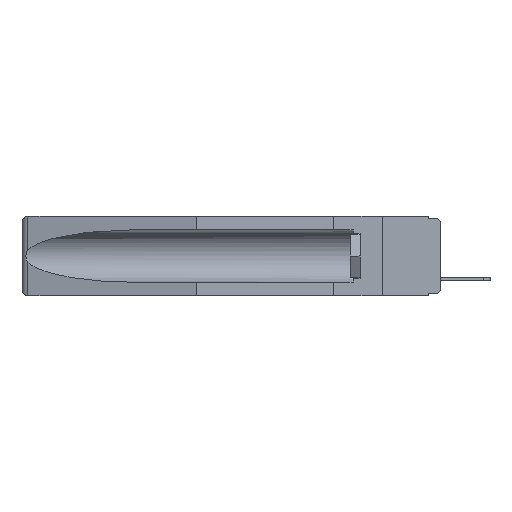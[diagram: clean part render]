
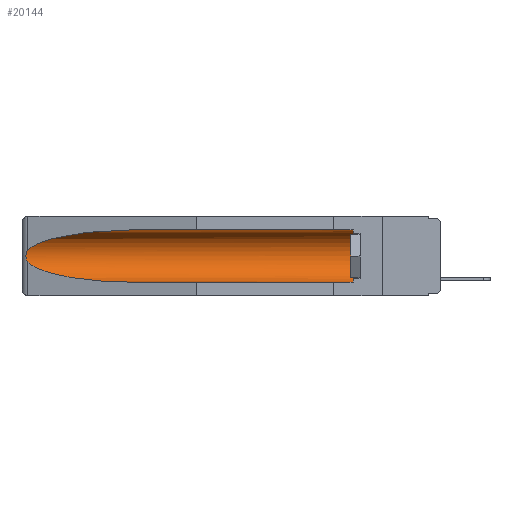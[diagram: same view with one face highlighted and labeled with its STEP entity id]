
A CAD part, left-side view. The second image highlights one B-rep face of the part: STEP entity #20144.
In plain terms, the highlighted cylindrical face has radius 2.857 mm (diameter 5.715 mm), a partial arc.
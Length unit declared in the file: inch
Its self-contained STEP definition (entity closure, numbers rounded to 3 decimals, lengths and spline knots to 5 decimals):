
#684 = DIRECTION ( 'NONE',  ( 0., 1., 0. ) ) ;
#697 = DIRECTION ( 'NONE',  ( 0., 1., 0. ) ) ;
#1230 = EDGE_CURVE ( 'NONE', #21232, #1581, #12304, .T. ) ;
#1581 = VERTEX_POINT ( 'NONE', #13792 ) ;
#2259 = AXIS2_PLACEMENT_3D ( 'NONE', #9138, #697, #20834 ) ;
#2445 = CARTESIAN_POINT ( 'NONE',  ( 0.155, -0.30754, -0.284 ) ) ;
#3760 = CARTESIAN_POINT ( 'NONE',  ( 0.155, 0.126, -0.1715 ) ) ;
#4679 = CARTESIAN_POINT ( 'NONE',  ( 0.2673, 1.5327, -0.16383 ) ) ;
#5197 = CARTESIAN_POINT ( 'NONE',  ( 0.26537, 1.52718, -0.14972 ) ) ;
#5404 = CARTESIAN_POINT ( 'NONE',  ( 0.21114, 1.30732, -0.059 ) ) ;
#5410 = VERTEX_POINT ( 'NONE', #13827 ) ;
#5419 = ORIENTED_EDGE ( 'NONE', *, *, #8624, .T. ) ;
#5649 = CARTESIAN_POINT ( 'NONE',  ( 0.26537, 1.52718, -0.19328 ) ) ;
#6218 = CARTESIAN_POINT ( 'NONE',  ( 0.26597, 1.52961, -0.15275 ) ) ;
#6237 = VERTEX_POINT ( 'NONE', #11287 ) ;
#6435 = CARTESIAN_POINT ( 'NONE',  ( 0.26655, 1.53094, -0.18657 ) ) ;
#7325 = EDGE_CURVE ( 'NONE', #20696, #21232, #14255, .T. ) ;
#7818 = ORIENTED_EDGE ( 'NONE', *, *, #16306, .T. ) ;
#7897 = CARTESIAN_POINT ( 'NONE',  ( 0.26537, 1.52718, -0.14972 ) ) ;
#8107 = CARTESIAN_POINT ( 'NONE',  ( 0.26537, 1.52718, -0.19328 ) ) ;
#8624 = EDGE_CURVE ( 'NONE', #11812, #5410, #18479, .T. ) ;
#8701 = ORIENTED_EDGE ( 'NONE', *, *, #7325, .T. ) ;
#8877 = CARTESIAN_POINT ( 'NONE',  ( 0.155, 1.07973, -0.284 ) ) ;
#9138 = CARTESIAN_POINT ( 'NONE',  ( 0.155, -0.30754, -0.1715 ) ) ;
#9272 = CARTESIAN_POINT ( 'NONE',  ( 0.155, -0.30754, -0.059 ) ) ;
#9832 = VECTOR ( 'NONE', #684, 39.37008 ) ;
#10224 = EDGE_LOOP ( 'NONE', ( #16617, #7818, #5419, #15835, #13134, #8701 ) ) ;
#11287 = CARTESIAN_POINT ( 'NONE',  ( 0.155, 0.126, -0.284 ) ) ;
#11518 = FACE_OUTER_BOUND ( 'NONE', #10224, .T. ) ;
#11812 = VERTEX_POINT ( 'NONE', #5649 ) ;
#12304 =( BOUNDED_CURVE ( )  B_SPLINE_CURVE ( 3, ( #18713, #5404, #17066, #5197 ),
 .UNSPECIFIED., .F., .F. ) 
 B_SPLINE_CURVE_WITH_KNOTS ( ( 4, 4 ),
 ( 4.71239, 6.08839 ),
 .UNSPECIFIED. ) 
 CURVE ( )  GEOMETRIC_REPRESENTATION_ITEM ( )  RATIONAL_B_SPLINE_CURVE ( ( 1., 0.848, 0.848, 1. ) ) 
 REPRESENTATION_ITEM ( '' )  );
#12768 = CARTESIAN_POINT ( 'NONE',  ( 0.155, 1.07973, -0.059 ) ) ;
#13134 = ORIENTED_EDGE ( 'NONE', *, *, #16993, .T. ) ;
#13758 = CIRCLE ( 'NONE', #17596, 0.1125 ) ;
#13792 = CARTESIAN_POINT ( 'NONE',  ( 0.26537, 1.52718, -0.14972 ) ) ;
#13809 = CARTESIAN_POINT ( 'NONE',  ( 0.21114, 1.30732, -0.284 ) ) ;
#13827 = CARTESIAN_POINT ( 'NONE',  ( 0.155, 1.07973, -0.284 ) ) ;
#13887 = CARTESIAN_POINT ( 'NONE',  ( 0.26537, 1.52718, -0.19328 ) ) ;
#14255 = LINE ( 'NONE', #9272, #9832 ) ;
#14655 = CARTESIAN_POINT ( 'NONE',  ( 0.26654, 1.53092, -0.15636 ) ) ;
#14728 = CARTESIAN_POINT ( 'NONE',  ( 0.2675, 1.53308, -0.17534 ) ) ;
#15417 = VECTOR ( 'NONE', #15780, 39.37008 ) ;
#15452 = EDGE_CURVE ( 'NONE', #6237, #5410, #19906, .T. ) ;
#15780 = DIRECTION ( 'NONE',  ( 0., 1., 0. ) ) ;
#15835 = ORIENTED_EDGE ( 'NONE', *, *, #15452, .F. ) ;
#16306 = EDGE_CURVE ( 'NONE', #1581, #11812, #16842, .T. ) ;
#16407 = CARTESIAN_POINT ( 'NONE',  ( 0.2673, 1.53269, -0.17917 ) ) ;
#16430 = CARTESIAN_POINT ( 'NONE',  ( 0.155, 0.126, -0.059 ) ) ;
#16617 = ORIENTED_EDGE ( 'NONE', *, *, #1230, .T. ) ;
#16842 = B_SPLINE_CURVE_WITH_KNOTS ( 'NONE', 3,
 ( #7897, #6218, #14655, #4679, #21405, #14728, #16407, #6435, #18102, #8107 ),
 .UNSPECIFIED., .F., .F.,
 ( 4, 2, 2, 2, 4 ),
 ( 0., 0.00029, 0.00058, 0.00087, 0.00117 ),
 .UNSPECIFIED. ) ;
#16993 = EDGE_CURVE ( 'NONE', #6237, #20696, #13758, .T. ) ;
#17066 = CARTESIAN_POINT ( 'NONE',  ( 0.25451, 1.48313, -0.09465 ) ) ;
#17596 = AXIS2_PLACEMENT_3D ( 'NONE', #3760, #18737, #18880 ) ;
#18102 = CARTESIAN_POINT ( 'NONE',  ( 0.26597, 1.5296, -0.19026 ) ) ;
#18479 =( BOUNDED_CURVE ( )  B_SPLINE_CURVE ( 3, ( #13887, #18814, #13809, #8877 ),
 .UNSPECIFIED., .F., .F. ) 
 B_SPLINE_CURVE_WITH_KNOTS ( ( 4, 4 ),
 ( 0.1948, 1.5708 ),
 .UNSPECIFIED. ) 
 CURVE ( )  GEOMETRIC_REPRESENTATION_ITEM ( )  RATIONAL_B_SPLINE_CURVE ( ( 1., 0.848, 0.848, 1. ) ) 
 REPRESENTATION_ITEM ( '' )  );
#18713 = CARTESIAN_POINT ( 'NONE',  ( 0.155, 1.07973, -0.059 ) ) ;
#18737 = DIRECTION ( 'NONE',  ( 0., -1., 0. ) ) ;
#18814 = CARTESIAN_POINT ( 'NONE',  ( 0.25451, 1.48313, -0.24835 ) ) ;
#18831 = CYLINDRICAL_SURFACE ( 'NONE', #2259, 0.1125 ) ;
#18880 = DIRECTION ( 'NONE',  ( 0., 0., 1. ) ) ;
#19906 = LINE ( 'NONE', #2445, #15417 ) ;
#20144 = ADVANCED_FACE ( 'NONE', ( #11518 ), #18831, .F. ) ;
#20696 = VERTEX_POINT ( 'NONE', #16430 ) ;
#20834 = DIRECTION ( 'NONE',  ( 0., 0., 1. ) ) ;
#21232 = VERTEX_POINT ( 'NONE', #12768 ) ;
#21405 = CARTESIAN_POINT ( 'NONE',  ( 0.2675, 1.53308, -0.16763 ) ) ;
